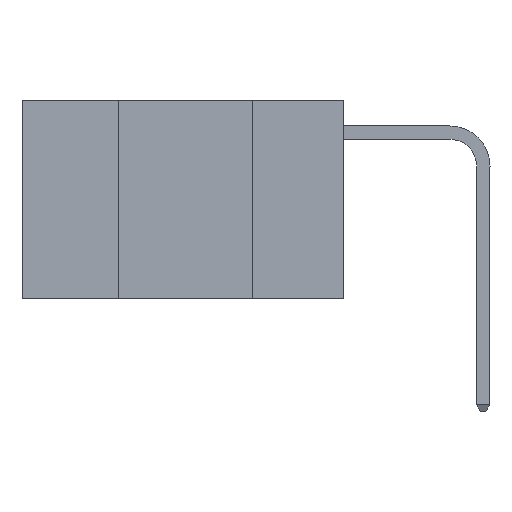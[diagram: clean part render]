
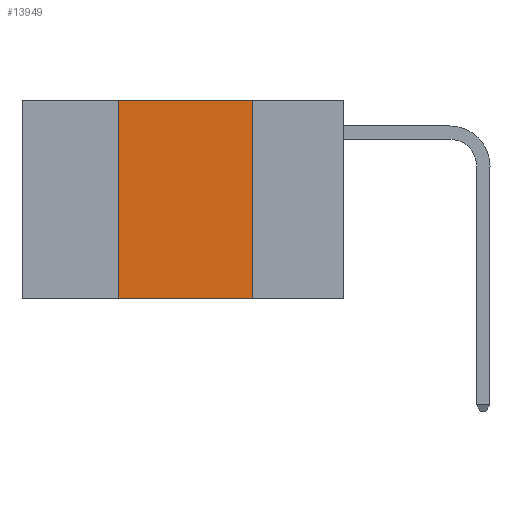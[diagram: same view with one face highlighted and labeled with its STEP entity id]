
A CAD part, left-side view. The second image highlights one B-rep face of the part: STEP entity #13949.
In plain terms, the highlighted planar face has unit normal (-1, 0, 0).
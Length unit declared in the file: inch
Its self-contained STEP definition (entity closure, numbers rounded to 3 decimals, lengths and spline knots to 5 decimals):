
#130 = VECTOR ( 'NONE', #14442, 39.37008 ) ;
#407 = CARTESIAN_POINT ( 'NONE',  ( 0., 0.17, 0. ) ) ;
#1031 = LINE ( 'NONE', #9155, #4383 ) ;
#1052 = CARTESIAN_POINT ( 'NONE',  ( 0., 0.42, -0.37 ) ) ;
#1366 = CARTESIAN_POINT ( 'NONE',  ( 0., 0.17, 0. ) ) ;
#3020 = VERTEX_POINT ( 'NONE', #6092 ) ;
#3221 = VECTOR ( 'NONE', #5342, 39.37008 ) ;
#3224 = EDGE_LOOP ( 'NONE', ( #5824, #5920, #5936, #6081 ) ) ;
#3603 = LINE ( 'NONE', #407, #3221 ) ;
#4383 = VECTOR ( 'NONE', #10360, 39.37008 ) ;
#4947 = DIRECTION ( 'NONE',  ( 0., 0., -1. ) ) ;
#5342 = DIRECTION ( 'NONE',  ( 0., 0., -1. ) ) ;
#5824 = ORIENTED_EDGE ( 'NONE', *, *, #11304, .F. ) ;
#5920 = ORIENTED_EDGE ( 'NONE', *, *, #5978, .F. ) ;
#5936 = ORIENTED_EDGE ( 'NONE', *, *, #10519, .F. ) ;
#5978 = EDGE_CURVE ( 'NONE', #3020, #9263, #11970, .T. ) ;
#6081 = ORIENTED_EDGE ( 'NONE', *, *, #9750, .T. ) ;
#6092 = CARTESIAN_POINT ( 'NONE',  ( 0., 0.42, 0. ) ) ;
#6664 = LINE ( 'NONE', #10252, #130 ) ;
#8486 = CARTESIAN_POINT ( 'NONE',  ( 0., 0.17, -0.37 ) ) ;
#9155 = CARTESIAN_POINT ( 'NONE',  ( 0., 0.6, -0.37 ) ) ;
#9263 = VERTEX_POINT ( 'NONE', #1366 ) ;
#9605 = PLANE ( 'NONE',  #12358 ) ;
#9750 = EDGE_CURVE ( 'NONE', #12276, #12458, #1031, .T. ) ;
#10252 = CARTESIAN_POINT ( 'NONE',  ( 0., 0.42, 0. ) ) ;
#10360 = DIRECTION ( 'NONE',  ( 0., -1., 0. ) ) ;
#10519 = EDGE_CURVE ( 'NONE', #12276, #3020, #6664, .T. ) ;
#10669 = FACE_OUTER_BOUND ( 'NONE', #3224, .T. ) ;
#11188 = VECTOR ( 'NONE', #13601, 39.37008 ) ;
#11304 = EDGE_CURVE ( 'NONE', #9263, #12458, #3603, .T. ) ;
#11923 = DIRECTION ( 'NONE',  ( 1., 0., 0. ) ) ;
#11970 = LINE ( 'NONE', #13696, #11188 ) ;
#12276 = VERTEX_POINT ( 'NONE', #1052 ) ;
#12358 = AXIS2_PLACEMENT_3D ( 'NONE', #14855, #11923, #4947 ) ;
#12458 = VERTEX_POINT ( 'NONE', #8486 ) ;
#13601 = DIRECTION ( 'NONE',  ( 0., -1., 0. ) ) ;
#13696 = CARTESIAN_POINT ( 'NONE',  ( 0., 0.6, 0. ) ) ;
#13949 = ADVANCED_FACE ( 'NONE', ( #10669 ), #9605, .F. ) ;
#14442 = DIRECTION ( 'NONE',  ( 0., 0., 1. ) ) ;
#14855 = CARTESIAN_POINT ( 'NONE',  ( 0., 0.6, 0. ) ) ;
